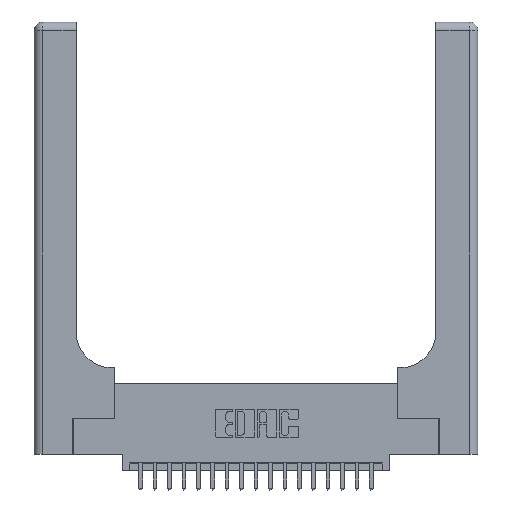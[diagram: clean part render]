
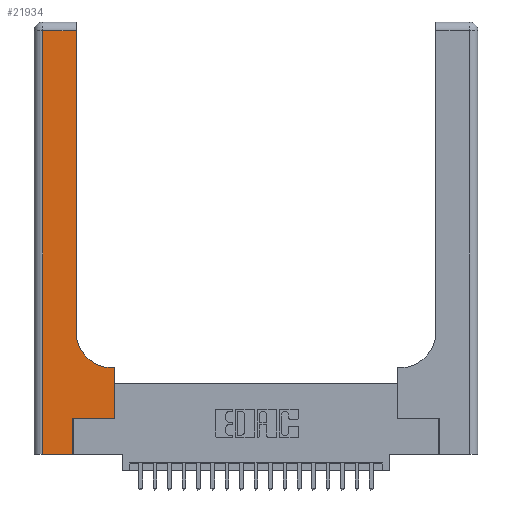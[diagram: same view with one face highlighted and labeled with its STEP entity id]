
A CAD part, top view. The second image highlights one B-rep face of the part: STEP entity #21934.
In plain terms, the highlighted planar face has unit normal (0, 0, 1).
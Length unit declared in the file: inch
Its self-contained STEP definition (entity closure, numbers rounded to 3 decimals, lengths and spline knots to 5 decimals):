
#189 = AXIS2_PLACEMENT_3D ( 'NONE', #5778, #17524, #15668 ) ;
#192 = CARTESIAN_POINT ( 'NONE',  ( 0.269, 0.25, 0.37 ) ) ;
#1571 = FACE_OUTER_BOUND ( 'NONE', #15572, .T. ) ;
#1682 = ORIENTED_EDGE ( 'NONE', *, *, #4513, .T. ) ;
#1788 = ORIENTED_EDGE ( 'NONE', *, *, #20725, .T. ) ;
#2401 = CARTESIAN_POINT ( 'NONE',  ( 0.5415, 0.6, 0.37 ) ) ;
#2596 = LINE ( 'NONE', #11615, #20146 ) ;
#2709 = ORIENTED_EDGE ( 'NONE', *, *, #17221, .T. ) ;
#3130 = DIRECTION ( 'NONE',  ( 0., 1., 0. ) ) ;
#3132 = CARTESIAN_POINT ( 'NONE',  ( 0.5585, 0.6, 0.37 ) ) ;
#3219 = LINE ( 'NONE', #7590, #12833 ) ;
#3474 = EDGE_CURVE ( 'NONE', #6288, #15074, #13752, .T. ) ;
#3669 = EDGE_CURVE ( 'NONE', #8811, #3706, #6845, .T. ) ;
#3706 = VERTEX_POINT ( 'NONE', #3132 ) ;
#4513 = EDGE_CURVE ( 'NONE', #3706, #6288, #10505, .T. ) ;
#4524 = VERTEX_POINT ( 'NONE', #192 ) ;
#4869 = EDGE_CURVE ( 'NONE', #17849, #4524, #2596, .T. ) ;
#5245 = CARTESIAN_POINT ( 'NONE',  ( 0.5585, 0.25, 0.37 ) ) ;
#5371 = EDGE_CURVE ( 'NONE', #15074, #13155, #16873, .T. ) ;
#5778 = CARTESIAN_POINT ( 'NONE',  ( 0.5415, 0.85, 0.37 ) ) ;
#5878 = VECTOR ( 'NONE', #7957, 39.37008 ) ;
#6288 = VERTEX_POINT ( 'NONE', #2401 ) ;
#6452 = CARTESIAN_POINT ( 'NONE',  ( 0.06, 3., 0.37 ) ) ;
#6845 = LINE ( 'NONE', #14727, #14815 ) ;
#6853 = DIRECTION ( 'NONE',  ( 1., 0., 0. ) ) ;
#7590 = CARTESIAN_POINT ( 'NONE',  ( 0., 2.94, 0.37 ) ) ;
#7957 = DIRECTION ( 'NONE',  ( 0., -1., 0. ) ) ;
#7977 = DIRECTION ( 'NONE',  ( -1., 0., 0. ) ) ;
#8811 = VERTEX_POINT ( 'NONE', #5245 ) ;
#9319 = ORIENTED_EDGE ( 'NONE', *, *, #3474, .T. ) ;
#9356 = LINE ( 'NONE', #6452, #5878 ) ;
#10297 = ORIENTED_EDGE ( 'NONE', *, *, #20607, .T. ) ;
#10505 = LINE ( 'NONE', #13607, #17417 ) ;
#10627 = CARTESIAN_POINT ( 'NONE',  ( 0.06, 2.94, 0.37 ) ) ;
#11615 = CARTESIAN_POINT ( 'NONE',  ( 0.269, 0., 0.37 ) ) ;
#11806 = ORIENTED_EDGE ( 'NONE', *, *, #4869, .T. ) ;
#11829 = DIRECTION ( 'NONE',  ( 1., 0., 0. ) ) ;
#11840 = ORIENTED_EDGE ( 'NONE', *, *, #5371, .T. ) ;
#12107 = CARTESIAN_POINT ( 'NONE',  ( 0.06, 0., 0.37 ) ) ;
#12726 = DIRECTION ( 'NONE',  ( -1., 0., 0. ) ) ;
#12818 = ORIENTED_EDGE ( 'NONE', *, *, #19885, .T. ) ;
#12819 = CARTESIAN_POINT ( 'NONE',  ( 0., 3., 0.37 ) ) ;
#12833 = VECTOR ( 'NONE', #12726, 39.37008 ) ;
#12897 = VECTOR ( 'NONE', #18311, 39.37008 ) ;
#13013 = VECTOR ( 'NONE', #11829, 39.37008 ) ;
#13021 = CARTESIAN_POINT ( 'NONE',  ( 0., 0., 0.37 ) ) ;
#13027 = PLANE ( 'NONE',  #21368 ) ;
#13111 = CARTESIAN_POINT ( 'NONE',  ( 0.2915, 0.85, 0.37 ) ) ;
#13155 = VERTEX_POINT ( 'NONE', #14426 ) ;
#13607 = CARTESIAN_POINT ( 'NONE',  ( 0.2915, 0.6, 0.37 ) ) ;
#13752 = CIRCLE ( 'NONE', #189, 0.25 ) ;
#13960 = CARTESIAN_POINT ( 'NONE',  ( 0.2915, 3., 0.37 ) ) ;
#14426 = CARTESIAN_POINT ( 'NONE',  ( 0.2915, 2.94, 0.37 ) ) ;
#14727 = CARTESIAN_POINT ( 'NONE',  ( 0.5585, 0.25, 0.37 ) ) ;
#14730 = DIRECTION ( 'NONE',  ( 0., 0., -1. ) ) ;
#14815 = VECTOR ( 'NONE', #21349, 39.37008 ) ;
#15074 = VERTEX_POINT ( 'NONE', #13111 ) ;
#15241 = DIRECTION ( 'NONE',  ( -1., 0., 0. ) ) ;
#15572 = EDGE_LOOP ( 'NONE', ( #11840, #10297, #1788, #12818, #11806, #2709, #17755, #1682, #9319 ) ) ;
#15668 = DIRECTION ( 'NONE',  ( 1., 0., 0. ) ) ;
#16873 = LINE ( 'NONE', #13960, #12897 ) ;
#17095 = VECTOR ( 'NONE', #6853, 39.37008 ) ;
#17221 = EDGE_CURVE ( 'NONE', #4524, #8811, #20692, .T. ) ;
#17417 = VECTOR ( 'NONE', #15241, 39.37008 ) ;
#17524 = DIRECTION ( 'NONE',  ( 0., 0., -1. ) ) ;
#17755 = ORIENTED_EDGE ( 'NONE', *, *, #3669, .T. ) ;
#17849 = VERTEX_POINT ( 'NONE', #19713 ) ;
#18095 = VERTEX_POINT ( 'NONE', #12107 ) ;
#18311 = DIRECTION ( 'NONE',  ( 0., 1., 0. ) ) ;
#18821 = CARTESIAN_POINT ( 'NONE',  ( 0.269, 0.25, 0.37 ) ) ;
#19599 = VERTEX_POINT ( 'NONE', #10627 ) ;
#19713 = CARTESIAN_POINT ( 'NONE',  ( 0.269, 0., 0.37 ) ) ;
#19885 = EDGE_CURVE ( 'NONE', #18095, #17849, #21625, .T. ) ;
#20146 = VECTOR ( 'NONE', #3130, 39.37008 ) ;
#20607 = EDGE_CURVE ( 'NONE', #13155, #19599, #3219, .T. ) ;
#20692 = LINE ( 'NONE', #18821, #13013 ) ;
#20725 = EDGE_CURVE ( 'NONE', #19599, #18095, #9356, .T. ) ;
#21349 = DIRECTION ( 'NONE',  ( 0., 1., 0. ) ) ;
#21368 = AXIS2_PLACEMENT_3D ( 'NONE', #12819, #14730, #7977 ) ;
#21625 = LINE ( 'NONE', #13021, #17095 ) ;
#21934 = ADVANCED_FACE ( 'NONE', ( #1571 ), #13027, .F. ) ;
